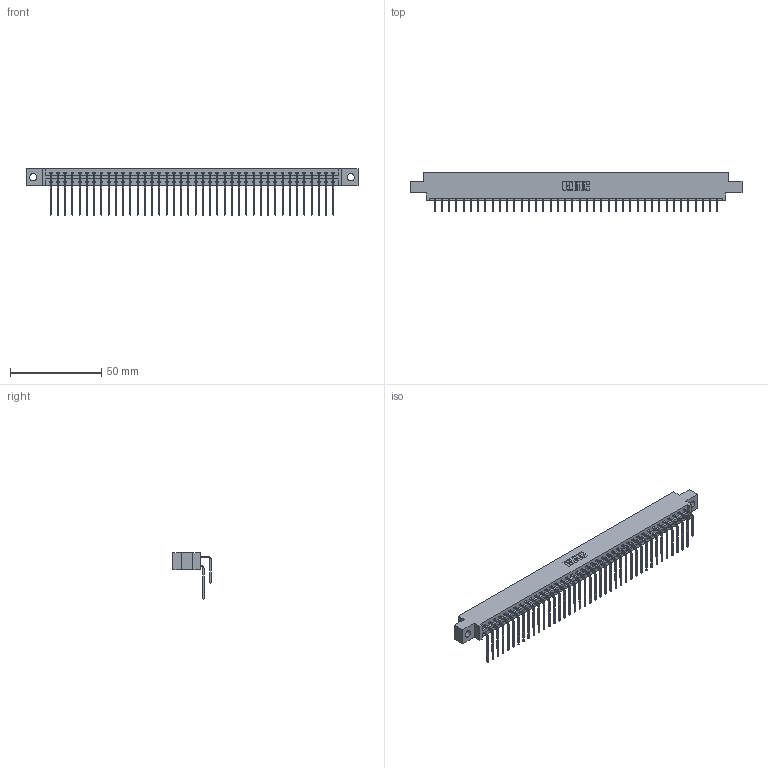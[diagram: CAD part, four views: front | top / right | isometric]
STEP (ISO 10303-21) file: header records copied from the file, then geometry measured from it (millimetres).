
FILE_DESCRIPTION (( 'STEP AP203' ), '1' );
FILE_NAME ('337-080-559-804.STEP', '2019-10-15T15:47:09', ( '' ), ( '' ), 'SwSTEP 2.0', 'SolidWorks 2016', '' );
FILE_SCHEMA (( 'CONFIG_CONTROL_DESIGN' ));
Length unit declared in the file: inch
Products named in the file (4): 345-292-001_558 559 Tail - 1; 345-292-001_559 Tail - 2; 337 Part_0.170 Offset - 0.156 Dia-TH; 337-080-559-804
Assembly tree (81 placements, depth 2):
  337-080-559-804
    337 Part_0.170 Offset - 0.156 Dia-TH
    345-292-001_558 559 Tail - 1  x40
    345-292-001_559 Tail - 2  x40
Bounding box: 181.51 x 20.9 x 25.53 mm (x, y, z)
Volume: 19358.3 mm3; surface area: 24087.7 mm2
Topology: 81 solids, 81 shells, 4598 faces, 13683 edges, 9014 vertices
Faces by surface type: plane 3274, cylinder 1324
Entity records: 33191 total; most frequent: CARTESIAN_POINT 5641, ORIENTED_EDGE 5526, DIRECTION 4783, EDGE_CURVE 2763, LINE 2595, VECTOR 2595, VERTEX_POINT 1838, AXIS2_PLACEMENT_3D 1094
